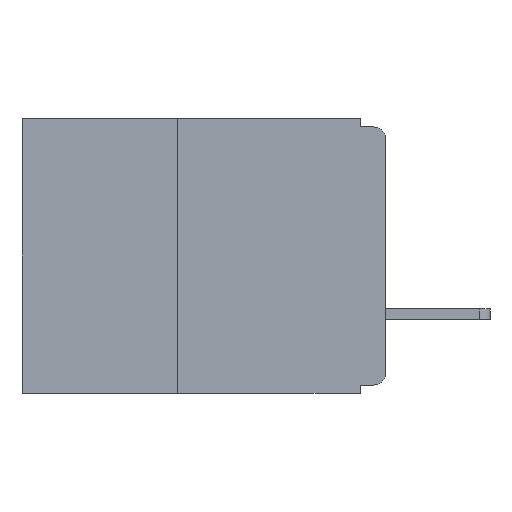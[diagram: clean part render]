
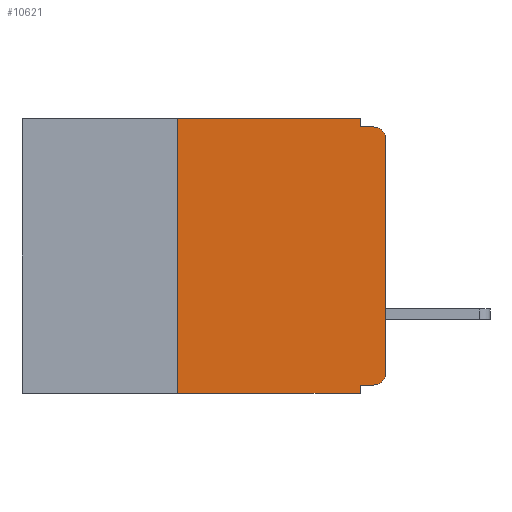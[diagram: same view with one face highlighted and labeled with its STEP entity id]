
A CAD part, left-side view. The second image highlights one B-rep face of the part: STEP entity #10621.
In plain terms, the highlighted planar face has unit normal (-1, 0, 0).
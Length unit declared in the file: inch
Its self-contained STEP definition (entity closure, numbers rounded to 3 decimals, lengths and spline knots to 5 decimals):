
#257 = AXIS2_PLACEMENT_3D ( 'NONE', #13513, #15095, #5616 ) ;
#288 = LINE ( 'NONE', #5540, #2305 ) ;
#455 = LINE ( 'NONE', #19382, #12675 ) ;
#481 = LINE ( 'NONE', #10749, #16351 ) ;
#569 = DIRECTION ( 'NONE',  ( 0., -1., 0. ) ) ;
#618 = EDGE_CURVE ( 'NONE', #12955, #16665, #12398, .T. ) ;
#779 = DIRECTION ( 'NONE',  ( 0., -1., 0. ) ) ;
#1489 = CARTESIAN_POINT ( 'NONE',  ( 0., 0., -0.01 ) ) ;
#2126 = AXIS2_PLACEMENT_3D ( 'NONE', #19903, #9318, #17708 ) ;
#2305 = VECTOR ( 'NONE', #779, 39.37008 ) ;
#2678 = CARTESIAN_POINT ( 'NONE',  ( 0., 0., 0. ) ) ;
#2822 = DIRECTION ( 'NONE',  ( 0., 1., 0. ) ) ;
#3118 = DIRECTION ( 'NONE',  ( 0., -1., 0. ) ) ;
#3188 = ORIENTED_EDGE ( 'NONE', *, *, #9217, .F. ) ;
#3535 = CARTESIAN_POINT ( 'NONE',  ( 0., 0.031, 0. ) ) ;
#4343 = VERTEX_POINT ( 'NONE', #12065 ) ;
#5050 = LINE ( 'NONE', #2678, #8765 ) ;
#5540 = CARTESIAN_POINT ( 'NONE',  ( 0., 0.437, 0. ) ) ;
#5550 = CARTESIAN_POINT ( 'NONE',  ( 0., 0.015, -0.32 ) ) ;
#5616 = DIRECTION ( 'NONE',  ( 0., 0., -1. ) ) ;
#5697 = VECTOR ( 'NONE', #17607, 39.37008 ) ;
#5761 = CARTESIAN_POINT ( 'NONE',  ( 0., 0.031, -0.33 ) ) ;
#5842 = ORIENTED_EDGE ( 'NONE', *, *, #7752, .T. ) ;
#5939 = CARTESIAN_POINT ( 'NONE',  ( 0., 0.031, -0.01 ) ) ;
#5947 = CARTESIAN_POINT ( 'NONE',  ( 0., 0.031, -0.33 ) ) ;
#6060 = EDGE_LOOP ( 'NONE', ( #11391, #18058, #16721, #3188, #12099, #14104, #5842, #17791, #11966, #14060 ) ) ;
#6196 = VERTEX_POINT ( 'NONE', #5939 ) ;
#6669 = EDGE_CURVE ( 'NONE', #14090, #13433, #8253, .T. ) ;
#6873 = CARTESIAN_POINT ( 'NONE',  ( 0., 0.25, -0.33 ) ) ;
#6920 = DIRECTION ( 'NONE',  ( -1., 0., 0. ) ) ;
#7724 = EDGE_CURVE ( 'NONE', #11008, #4343, #13157, .T. ) ;
#7752 = EDGE_CURVE ( 'NONE', #14090, #10773, #455, .T. ) ;
#7995 = EDGE_CURVE ( 'NONE', #12955, #19168, #481, .T. ) ;
#8253 = LINE ( 'NONE', #18378, #11976 ) ;
#8765 = VECTOR ( 'NONE', #15298, 39.37008 ) ;
#9217 = EDGE_CURVE ( 'NONE', #19236, #6196, #9907, .T. ) ;
#9318 = DIRECTION ( 'NONE',  ( -1., 0., 0. ) ) ;
#9907 = LINE ( 'NONE', #3535, #5697 ) ;
#10315 = CARTESIAN_POINT ( 'NONE',  ( 0., 0.25, 0. ) ) ;
#10550 = DIRECTION ( 'NONE',  ( 0., 0., -1. ) ) ;
#10599 = LINE ( 'NONE', #1489, #18358 ) ;
#10621 = ADVANCED_FACE ( 'NONE', ( #17667 ), #11922, .F. ) ;
#10654 = DIRECTION ( 'NONE',  ( 0., 0., 1. ) ) ;
#10749 = CARTESIAN_POINT ( 'NONE',  ( 0., 0., -0.32 ) ) ;
#10773 = VERTEX_POINT ( 'NONE', #5947 ) ;
#10793 = EDGE_CURVE ( 'NONE', #6196, #4343, #10599, .T. ) ;
#10966 = CARTESIAN_POINT ( 'NONE',  ( 0., 0.031, 0. ) ) ;
#11008 = VERTEX_POINT ( 'NONE', #16162 ) ;
#11391 = ORIENTED_EDGE ( 'NONE', *, *, #19876, .T. ) ;
#11922 = PLANE ( 'NONE',  #257 ) ;
#11966 = ORIENTED_EDGE ( 'NONE', *, *, #7995, .F. ) ;
#11976 = VECTOR ( 'NONE', #10654, 39.37008 ) ;
#12065 = CARTESIAN_POINT ( 'NONE',  ( 0., 0.015, -0.01 ) ) ;
#12099 = ORIENTED_EDGE ( 'NONE', *, *, #19477, .F. ) ;
#12398 = CIRCLE ( 'NONE', #2126, 0.015 ) ;
#12675 = VECTOR ( 'NONE', #569, 39.37008 ) ;
#12955 = VERTEX_POINT ( 'NONE', #5550 ) ;
#13157 = CIRCLE ( 'NONE', #14221, 0.015 ) ;
#13433 = VERTEX_POINT ( 'NONE', #10315 ) ;
#13513 = CARTESIAN_POINT ( 'NONE',  ( 0., 0.437, 0. ) ) ;
#14060 = ORIENTED_EDGE ( 'NONE', *, *, #618, .T. ) ;
#14090 = VERTEX_POINT ( 'NONE', #6873 ) ;
#14104 = ORIENTED_EDGE ( 'NONE', *, *, #6669, .F. ) ;
#14221 = AXIS2_PLACEMENT_3D ( 'NONE', #16370, #6920, #17885 ) ;
#15095 = DIRECTION ( 'NONE',  ( 1., 0., 0. ) ) ;
#15158 = CARTESIAN_POINT ( 'NONE',  ( 0., 0., -0.305 ) ) ;
#15298 = DIRECTION ( 'NONE',  ( 0., 0., 1. ) ) ;
#16162 = CARTESIAN_POINT ( 'NONE',  ( 0., 0., -0.025 ) ) ;
#16202 = EDGE_CURVE ( 'NONE', #19168, #10773, #17259, .T. ) ;
#16351 = VECTOR ( 'NONE', #2822, 39.37008 ) ;
#16370 = CARTESIAN_POINT ( 'NONE',  ( 0., 0.015, -0.025 ) ) ;
#16665 = VERTEX_POINT ( 'NONE', #15158 ) ;
#16721 = ORIENTED_EDGE ( 'NONE', *, *, #10793, .F. ) ;
#16791 = VECTOR ( 'NONE', #10550, 39.37008 ) ;
#17025 = CARTESIAN_POINT ( 'NONE',  ( 0., 0.031, -0.32 ) ) ;
#17259 = LINE ( 'NONE', #5761, #16791 ) ;
#17607 = DIRECTION ( 'NONE',  ( 0., 0., -1. ) ) ;
#17667 = FACE_OUTER_BOUND ( 'NONE', #6060, .T. ) ;
#17708 = DIRECTION ( 'NONE',  ( 0., 0., -1. ) ) ;
#17791 = ORIENTED_EDGE ( 'NONE', *, *, #16202, .F. ) ;
#17885 = DIRECTION ( 'NONE',  ( 0., 0., -1. ) ) ;
#18058 = ORIENTED_EDGE ( 'NONE', *, *, #7724, .T. ) ;
#18358 = VECTOR ( 'NONE', #3118, 39.37008 ) ;
#18378 = CARTESIAN_POINT ( 'NONE',  ( 0., 0.25, -0.33 ) ) ;
#19168 = VERTEX_POINT ( 'NONE', #17025 ) ;
#19236 = VERTEX_POINT ( 'NONE', #10966 ) ;
#19382 = CARTESIAN_POINT ( 'NONE',  ( 0., 0.437, -0.33 ) ) ;
#19477 = EDGE_CURVE ( 'NONE', #13433, #19236, #288, .T. ) ;
#19876 = EDGE_CURVE ( 'NONE', #16665, #11008, #5050, .T. ) ;
#19903 = CARTESIAN_POINT ( 'NONE',  ( 0., 0.015, -0.305 ) ) ;
